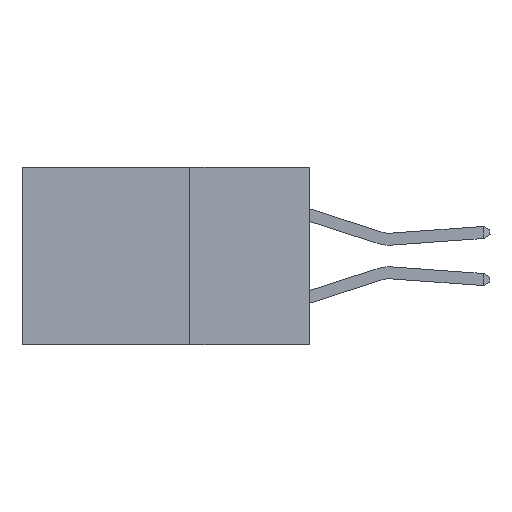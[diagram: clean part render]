
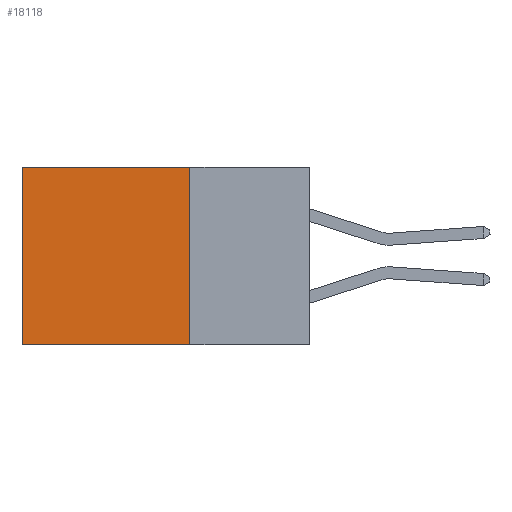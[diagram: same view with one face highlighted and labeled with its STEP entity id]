
A CAD part, left-side view. The second image highlights one B-rep face of the part: STEP entity #18118.
In plain terms, the highlighted planar face has unit normal (-1, 0, 0).
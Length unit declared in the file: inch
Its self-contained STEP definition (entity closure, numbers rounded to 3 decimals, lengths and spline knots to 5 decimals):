
#918 = VECTOR ( 'NONE', #11662, 39.37008 ) ;
#2345 = LINE ( 'NONE', #14458, #5448 ) ;
#2910 = EDGE_CURVE ( 'NONE', #16336, #13558, #7991, .T. ) ;
#3690 = LINE ( 'NONE', #6882, #918 ) ;
#4677 = CARTESIAN_POINT ( 'NONE',  ( 0.298, 0.25, 0. ) ) ;
#5448 = VECTOR ( 'NONE', #27689, 39.37008 ) ;
#6119 = LINE ( 'NONE', #4677, #25188 ) ;
#6347 = CARTESIAN_POINT ( 'NONE',  ( 0.298, 0.25, 0. ) ) ;
#6882 = CARTESIAN_POINT ( 'NONE',  ( 0.298, 0.25, -0.37 ) ) ;
#7263 = DIRECTION ( 'NONE',  ( 0., 0., -1. ) ) ;
#7301 = VECTOR ( 'NONE', #21663, 39.37008 ) ;
#7799 = VERTEX_POINT ( 'NONE', #9327 ) ;
#7991 = LINE ( 'NONE', #17386, #7301 ) ;
#8660 = DIRECTION ( 'NONE',  ( 0., 0., -1. ) ) ;
#8763 = DIRECTION ( 'NONE',  ( 1., 0., 0. ) ) ;
#9327 = CARTESIAN_POINT ( 'NONE',  ( 0.298, 0.25, 0. ) ) ;
#9506 = EDGE_CURVE ( 'NONE', #7799, #16336, #2345, .T. ) ;
#9978 = ORIENTED_EDGE ( 'NONE', *, *, #2910, .T. ) ;
#11662 = DIRECTION ( 'NONE',  ( 0., 1., 0. ) ) ;
#13558 = VERTEX_POINT ( 'NONE', #13940 ) ;
#13940 = CARTESIAN_POINT ( 'NONE',  ( 0.298, 0.6, -0.37 ) ) ;
#14458 = CARTESIAN_POINT ( 'NONE',  ( 0.298, 0.25, 0. ) ) ;
#14964 = VERTEX_POINT ( 'NONE', #26474 ) ;
#15532 = ORIENTED_EDGE ( 'NONE', *, *, #25513, .F. ) ;
#16336 = VERTEX_POINT ( 'NONE', #25074 ) ;
#16626 = EDGE_LOOP ( 'NONE', ( #9978, #15532, #28564, #25507 ) ) ;
#16790 = AXIS2_PLACEMENT_3D ( 'NONE', #6347, #8763, #8660 ) ;
#17386 = CARTESIAN_POINT ( 'NONE',  ( 0.298, 0.6, 0. ) ) ;
#17590 = PLANE ( 'NONE',  #16790 ) ;
#18118 = ADVANCED_FACE ( 'NONE', ( #20535 ), #17590, .F. ) ;
#20535 = FACE_OUTER_BOUND ( 'NONE', #16626, .T. ) ;
#21663 = DIRECTION ( 'NONE',  ( 0., 0., -1. ) ) ;
#25074 = CARTESIAN_POINT ( 'NONE',  ( 0.298, 0.6, 0. ) ) ;
#25188 = VECTOR ( 'NONE', #7263, 39.37008 ) ;
#25507 = ORIENTED_EDGE ( 'NONE', *, *, #9506, .T. ) ;
#25513 = EDGE_CURVE ( 'NONE', #14964, #13558, #3690, .T. ) ;
#25556 = EDGE_CURVE ( 'NONE', #7799, #14964, #6119, .T. ) ;
#26474 = CARTESIAN_POINT ( 'NONE',  ( 0.298, 0.25, -0.37 ) ) ;
#27689 = DIRECTION ( 'NONE',  ( 0., 1., 0. ) ) ;
#28564 = ORIENTED_EDGE ( 'NONE', *, *, #25556, .F. ) ;
